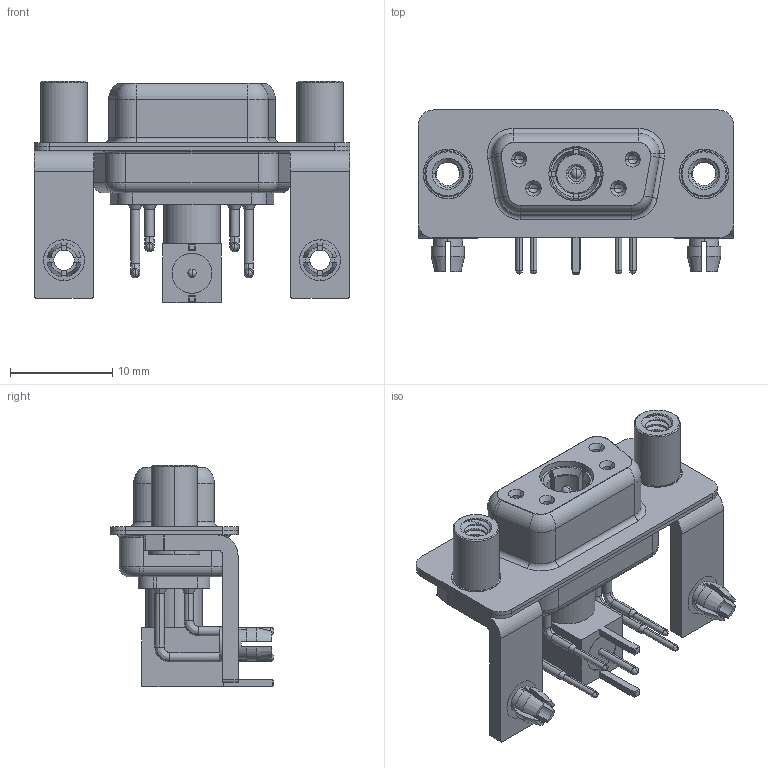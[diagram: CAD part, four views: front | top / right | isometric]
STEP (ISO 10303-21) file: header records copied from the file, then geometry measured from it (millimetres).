
FILE_DESCRIPTION (( 'STEP AP203' ), '1' );
FILE_NAME ('630-5W1-240-7T5.STEP', '2022-05-27T07:58:55', ( '' ), ( '' ), 'SwSTEP 2.0', 'SolidWorks 2020', '' );
FILE_SCHEMA (( 'CONFIG_CONTROL_DESIGN' ));
Length unit declared in the file: millimetre
Products named in the file (16): 630Combo Threaded Standoff_5; 630Combo Contact Row 2; Locking Collar; 630Combo Shell Front_09 Contacts; 630-5W1-240-7T5; 630Combo Board Lock; Co-Ax Plug Assy_RA; 630Combo Contact Row 1; Pin_RA; 630Combo Housing_5W1; 630Combo Stabilizer Bracket; RA Back Shell; 630Combo Shell Rear_09 Contacts; Insulator Pin_Straight PC Tail; Insulator RA Pin; Co-Ax Plug_RA PC Tail
Assembly tree (20 placements, depth 3):
  630-5W1-240-7T5
    630Combo Housing_5W1
    630Combo Shell Front_09 Contacts
    630Combo Shell Rear_09 Contacts
    630Combo Stabilizer Bracket  x2
    630Combo Board Lock  x2
    630Combo Threaded Standoff_5  x2
    Co-Ax Plug Assy_RA
      Co-Ax Plug_RA PC Tail
      Insulator Pin_Straight PC Tail
      Pin_RA
      Locking Collar
      RA Back Shell
      Insulator RA Pin
    630Combo Contact Row 1  x2
    630Combo Contact Row 2  x2
Bounding box: 30.8 x 16 x 21.61 mm (x, y, z)
Volume: 2404.1 mm3; surface area: 6136.7 mm2
Topology: 19 solids, 19 shells, 839 faces, 2110 edges, 1336 vertices
Faces by surface type: cylinder 386, plane 264, cone 99, torus 63, bspline 23, sphere 4
Entity records: 22862 total; most frequent: CARTESIAN_POINT 5719, DIRECTION 3407, ORIENTED_EDGE 3106, EDGE_CURVE 1553, AXIS2_PLACEMENT_3D 1365, VERTEX_POINT 989, EDGE_LOOP 718, CIRCLE 717
